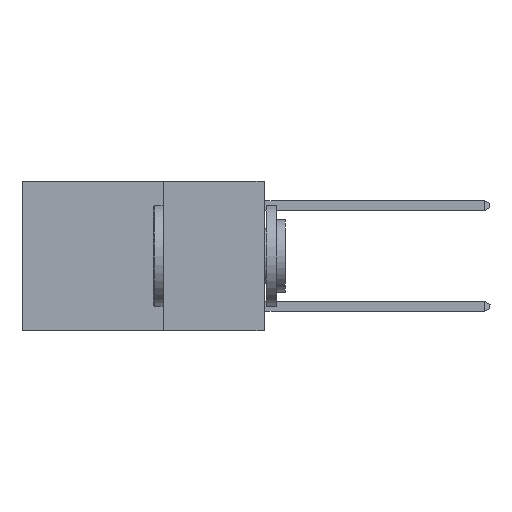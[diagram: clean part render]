
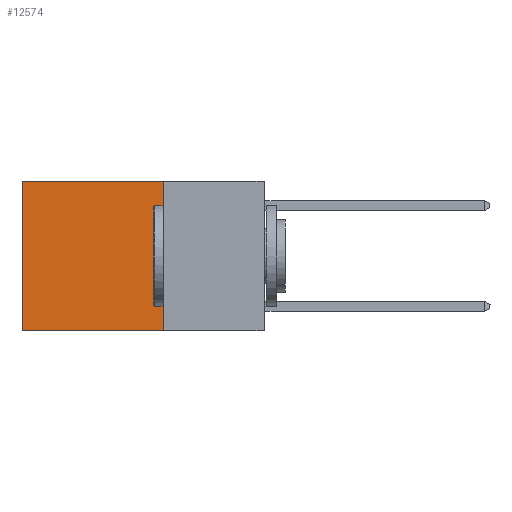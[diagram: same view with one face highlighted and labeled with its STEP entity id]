
A CAD part, left-side view. The second image highlights one B-rep face of the part: STEP entity #12574.
In plain terms, the highlighted planar face has unit normal (-1, 0, 0).
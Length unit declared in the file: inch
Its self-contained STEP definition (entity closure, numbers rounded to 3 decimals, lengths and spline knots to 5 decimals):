
#153 = VECTOR ( 'NONE', #20789, 39.37008 ) ;
#1436 = CARTESIAN_POINT ( 'NONE',  ( 0.2625, 0.25, 0. ) ) ;
#1847 = CARTESIAN_POINT ( 'NONE',  ( 0.2625, 0.6, 0. ) ) ;
#2283 = EDGE_CURVE ( 'NONE', #14708, #4279, #5500, .T. ) ;
#3358 = CARTESIAN_POINT ( 'NONE',  ( 0.2625, 0.25, 0. ) ) ;
#3455 = DIRECTION ( 'NONE',  ( 0., 0., -1. ) ) ;
#3949 = CARTESIAN_POINT ( 'NONE',  ( 0.2625, 0.6, -0.37 ) ) ;
#3965 = ORIENTED_EDGE ( 'NONE', *, *, #2283, .T. ) ;
#4279 = VERTEX_POINT ( 'NONE', #1847 ) ;
#5500 = LINE ( 'NONE', #25842, #20264 ) ;
#5984 = ORIENTED_EDGE ( 'NONE', *, *, #21796, .F. ) ;
#7476 = EDGE_CURVE ( 'NONE', #4279, #18120, #9645, .T. ) ;
#8168 = FACE_OUTER_BOUND ( 'NONE', #9065, .T. ) ;
#8844 = PLANE ( 'NONE',  #23260 ) ;
#9065 = EDGE_LOOP ( 'NONE', ( #13011, #12111, #5984, #3965 ) ) ;
#9645 = LINE ( 'NONE', #16767, #153 ) ;
#10879 = DIRECTION ( 'NONE',  ( 0., 0., -1. ) ) ;
#11328 = DIRECTION ( 'NONE',  ( 0., 1., 0. ) ) ;
#12111 = ORIENTED_EDGE ( 'NONE', *, *, #12701, .F. ) ;
#12574 = ADVANCED_FACE ( 'NONE', ( #8168 ), #8844, .F. ) ;
#12701 = EDGE_CURVE ( 'NONE', #17142, #18120, #21053, .T. ) ;
#13011 = ORIENTED_EDGE ( 'NONE', *, *, #7476, .T. ) ;
#14141 = LINE ( 'NONE', #1436, #24783 ) ;
#14708 = VERTEX_POINT ( 'NONE', #3358 ) ;
#14853 = CARTESIAN_POINT ( 'NONE',  ( 0.2625, 0.25, 0. ) ) ;
#16767 = CARTESIAN_POINT ( 'NONE',  ( 0.2625, 0.6, 0. ) ) ;
#17142 = VERTEX_POINT ( 'NONE', #23362 ) ;
#18120 = VERTEX_POINT ( 'NONE', #3949 ) ;
#20264 = VECTOR ( 'NONE', #21849, 39.37008 ) ;
#20424 = VECTOR ( 'NONE', #11328, 39.37008 ) ;
#20789 = DIRECTION ( 'NONE',  ( 0., 0., -1. ) ) ;
#21053 = LINE ( 'NONE', #25337, #20424 ) ;
#21796 = EDGE_CURVE ( 'NONE', #14708, #17142, #14141, .T. ) ;
#21849 = DIRECTION ( 'NONE',  ( 0., 1., 0. ) ) ;
#22917 = DIRECTION ( 'NONE',  ( 1., 0., 0. ) ) ;
#23260 = AXIS2_PLACEMENT_3D ( 'NONE', #14853, #22917, #10879 ) ;
#23362 = CARTESIAN_POINT ( 'NONE',  ( 0.2625, 0.25, -0.37 ) ) ;
#24783 = VECTOR ( 'NONE', #3455, 39.37008 ) ;
#25337 = CARTESIAN_POINT ( 'NONE',  ( 0.2625, 0.25, -0.37 ) ) ;
#25842 = CARTESIAN_POINT ( 'NONE',  ( 0.2625, 0.25, 0. ) ) ;
